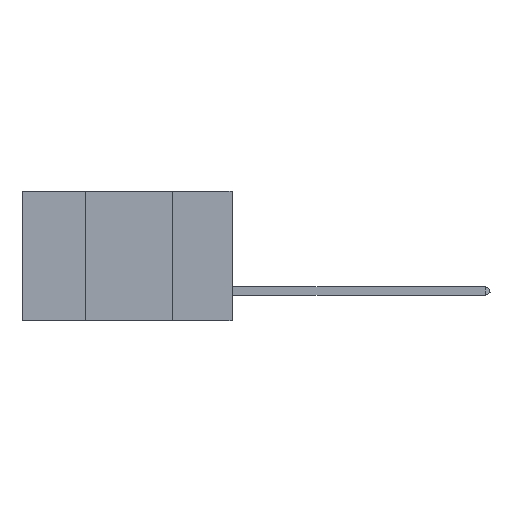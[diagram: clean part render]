
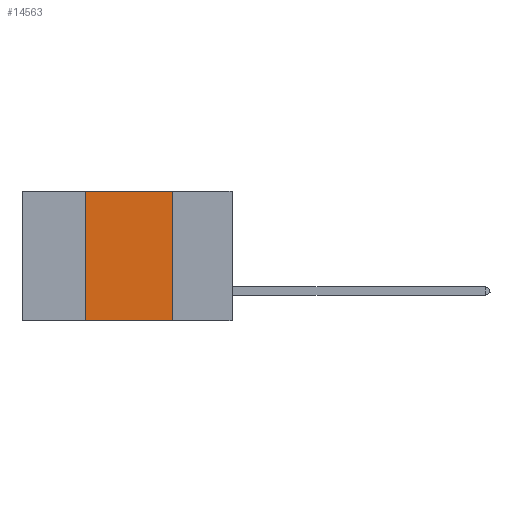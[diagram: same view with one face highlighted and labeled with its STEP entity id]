
A CAD part, left-side view. The second image highlights one B-rep face of the part: STEP entity #14563.
In plain terms, the highlighted planar face has unit normal (-1, 0, 0).
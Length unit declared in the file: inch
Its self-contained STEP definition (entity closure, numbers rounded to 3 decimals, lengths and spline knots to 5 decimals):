
#1971 = CARTESIAN_POINT ( 'NONE',  ( 0., 0.42, -0.37 ) ) ;
#3428 = LINE ( 'NONE', #9232, #18164 ) ;
#3727 = DIRECTION ( 'NONE',  ( 0., 0., -1. ) ) ;
#4569 = ORIENTED_EDGE ( 'NONE', *, *, #16938, .F. ) ;
#4862 = CARTESIAN_POINT ( 'NONE',  ( 0., 0.6, 0. ) ) ;
#5023 = DIRECTION ( 'NONE',  ( 0., 0., -1. ) ) ;
#5336 = DIRECTION ( 'NONE',  ( 0., 0., 1. ) ) ;
#5383 = CARTESIAN_POINT ( 'NONE',  ( 0., 0.17, 0. ) ) ;
#5705 = ORIENTED_EDGE ( 'NONE', *, *, #7299, .F. ) ;
#6436 = VERTEX_POINT ( 'NONE', #1971 ) ;
#6763 = VECTOR ( 'NONE', #5023, 39.37008 ) ;
#7299 = EDGE_CURVE ( 'NONE', #16585, #17961, #8416, .T. ) ;
#7481 = ORIENTED_EDGE ( 'NONE', *, *, #8598, .T. ) ;
#7855 = DIRECTION ( 'NONE',  ( 0., -1., 0. ) ) ;
#8353 = CARTESIAN_POINT ( 'NONE',  ( 0., 0.42, 0. ) ) ;
#8416 = LINE ( 'NONE', #9106, #6763 ) ;
#8598 = EDGE_CURVE ( 'NONE', #6436, #17961, #10034, .T. ) ;
#9106 = CARTESIAN_POINT ( 'NONE',  ( 0., 0.17, 0. ) ) ;
#9232 = CARTESIAN_POINT ( 'NONE',  ( 0., 0.6, 0. ) ) ;
#9290 = PLANE ( 'NONE',  #16752 ) ;
#10034 = LINE ( 'NONE', #10460, #16557 ) ;
#10460 = CARTESIAN_POINT ( 'NONE',  ( 0., 0.6, -0.37 ) ) ;
#12626 = VECTOR ( 'NONE', #5336, 39.37008 ) ;
#12699 = EDGE_LOOP ( 'NONE', ( #5705, #4569, #17363, #7481 ) ) ;
#14513 = LINE ( 'NONE', #8353, #12626 ) ;
#14563 = ADVANCED_FACE ( 'NONE', ( #16139 ), #9290, .F. ) ;
#14947 = CARTESIAN_POINT ( 'NONE',  ( 0., 0.17, -0.37 ) ) ;
#15229 = EDGE_CURVE ( 'NONE', #6436, #18583, #14513, .T. ) ;
#15694 = DIRECTION ( 'NONE',  ( 1., 0., 0. ) ) ;
#16139 = FACE_OUTER_BOUND ( 'NONE', #12699, .T. ) ;
#16487 = CARTESIAN_POINT ( 'NONE',  ( 0., 0.42, 0. ) ) ;
#16557 = VECTOR ( 'NONE', #19370, 39.37008 ) ;
#16585 = VERTEX_POINT ( 'NONE', #5383 ) ;
#16752 = AXIS2_PLACEMENT_3D ( 'NONE', #4862, #15694, #3727 ) ;
#16938 = EDGE_CURVE ( 'NONE', #18583, #16585, #3428, .T. ) ;
#17363 = ORIENTED_EDGE ( 'NONE', *, *, #15229, .F. ) ;
#17961 = VERTEX_POINT ( 'NONE', #14947 ) ;
#18164 = VECTOR ( 'NONE', #7855, 39.37008 ) ;
#18583 = VERTEX_POINT ( 'NONE', #16487 ) ;
#19370 = DIRECTION ( 'NONE',  ( 0., -1., 0. ) ) ;
